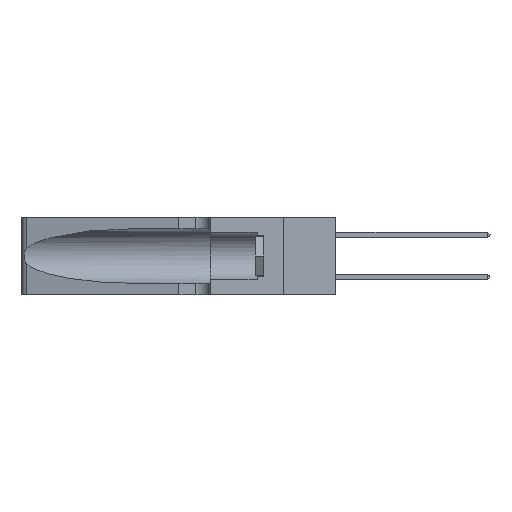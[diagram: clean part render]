
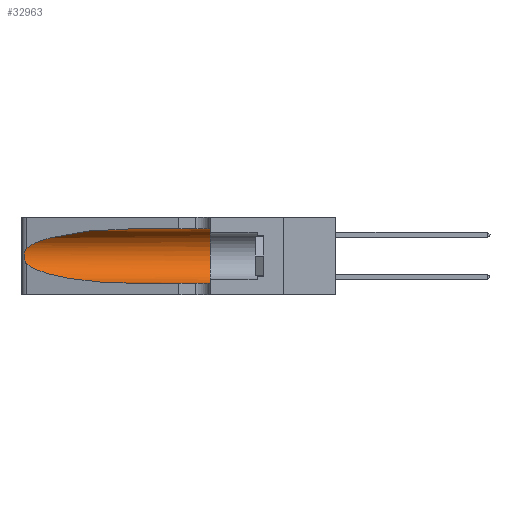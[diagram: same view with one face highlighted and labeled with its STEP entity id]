
A CAD part, left-side view. The second image highlights one B-rep face of the part: STEP entity #32963.
In plain terms, the highlighted cylindrical face has radius 3.308 mm (diameter 6.617 mm), a partial arc.
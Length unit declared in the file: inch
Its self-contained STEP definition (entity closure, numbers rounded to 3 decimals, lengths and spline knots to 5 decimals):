
#374 = EDGE_CURVE ( 'NONE', #2615, #19318, #17843, .T. ) ;
#410 = CARTESIAN_POINT ( 'NONE',  ( 0.18966, 0.96281, 0.05475 ) ) ;
#837 =( BOUNDED_CURVE ( )  B_SPLINE_CURVE ( 3, ( #3240, #30470, #410, #13938 ),
 .UNSPECIFIED., .F., .F. ) 
 B_SPLINE_CURVE_WITH_KNOTS ( ( 4, 4 ),
 ( 3.44316, 4.71239 ),
 .UNSPECIFIED. ) 
 CURVE ( )  GEOMETRIC_REPRESENTATION_ITEM ( )  RATIONAL_B_SPLINE_CURVE ( ( 1., 0.87, 0.87, 1. ) ) 
 REPRESENTATION_ITEM ( '' )  );
#1747 = CARTESIAN_POINT ( 'NONE',  ( 0.25487, 1.22718, 0.14631 ) ) ;
#2615 = VERTEX_POINT ( 'NONE', #20780 ) ;
#2907 = ORIENTED_EDGE ( 'NONE', *, *, #21805, .T. ) ;
#3240 = CARTESIAN_POINT ( 'NONE',  ( 0.25487, 1.22718, 0.14631 ) ) ;
#3848 = ORIENTED_EDGE ( 'NONE', *, *, #15714, .T. ) ;
#4164 = ORIENTED_EDGE ( 'NONE', *, *, #374, .F. ) ;
#4166 = CARTESIAN_POINT ( 'NONE',  ( 0.25555, 1.22994, 0.2215 ) ) ;
#4283 = CARTESIAN_POINT ( 'NONE',  ( 0.25639, 1.23186, 0.15144 ) ) ;
#5336 = CARTESIAN_POINT ( 'NONE',  ( 0.1305, 1.61858, 0.31525 ) ) ;
#5364 = LINE ( 'NONE', #10373, #8414 ) ;
#5399 = CARTESIAN_POINT ( 'NONE',  ( 0.1305, 0.72297, 0.31525 ) ) ;
#5685 = VERTEX_POINT ( 'NONE', #25413 ) ;
#6940 = CARTESIAN_POINT ( 'NONE',  ( 0.25555, 1.22993, 0.14849 ) ) ;
#7965 = LINE ( 'NONE', #5336, #10157 ) ;
#8414 = VECTOR ( 'NONE', #18704, 39.37008 ) ;
#8447 = CARTESIAN_POINT ( 'NONE',  ( 0.25487, 1.22718, 0.22369 ) ) ;
#10157 = VECTOR ( 'NONE', #19144, 39.37008 ) ;
#10373 = CARTESIAN_POINT ( 'NONE',  ( 0.1305, 1.61858, 0.05475 ) ) ;
#11327 = CARTESIAN_POINT ( 'NONE',  ( 0.1305, 0.35, 0.05475 ) ) ;
#11475 = AXIS2_PLACEMENT_3D ( 'NONE', #22306, #22669, #14192 ) ;
#11914 = B_SPLINE_CURVE_WITH_KNOTS ( 'NONE', 3,
 ( #15101, #4166, #31784, #15339, #20682, #23367, #12471, #34529, #17951, #18066, #20565, #4283, #6940, #1747 ),
 .UNSPECIFIED., .F., .F.,
 ( 4, 2, 2, 2, 2, 2, 4 ),
 ( 0., 0.00027, 0.00053, 0.00107, 0.0016, 0.00187, 0.00214 ),
 .UNSPECIFIED. ) ;
#12471 = CARTESIAN_POINT ( 'NONE',  ( 0.26075, 1.23896, 0.19203 ) ) ;
#13393 = CARTESIAN_POINT ( 'NONE',  ( 0.1305, 0.72297, 0.31525 ) ) ;
#13938 = CARTESIAN_POINT ( 'NONE',  ( 0.1305, 0.72297, 0.05475 ) ) ;
#14192 = DIRECTION ( 'NONE',  ( 0., 0., -1. ) ) ;
#14695 = CARTESIAN_POINT ( 'NONE',  ( 0.25487, 1.22718, 0.22369 ) ) ;
#15101 = CARTESIAN_POINT ( 'NONE',  ( 0.25487, 1.22718, 0.22369 ) ) ;
#15339 = CARTESIAN_POINT ( 'NONE',  ( 0.25787, 1.23484, 0.2124 ) ) ;
#15714 = EDGE_CURVE ( 'NONE', #22904, #5685, #11914, .T. ) ;
#17843 = CIRCLE ( 'NONE', #31739, 0.13025 ) ;
#17951 = CARTESIAN_POINT ( 'NONE',  ( 0.26017, 1.23833, 0.17102 ) ) ;
#18066 = CARTESIAN_POINT ( 'NONE',  ( 0.25856, 1.23593, 0.16098 ) ) ;
#18132 = CYLINDRICAL_SURFACE ( 'NONE', #11475, 0.13025 ) ;
#18673 = EDGE_CURVE ( 'NONE', #35394, #2615, #7965, .T. ) ;
#18704 = DIRECTION ( 'NONE',  ( 0., -1., 0. ) ) ;
#19015 = FACE_OUTER_BOUND ( 'NONE', #28119, .T. ) ;
#19144 = DIRECTION ( 'NONE',  ( 0., -1., 0. ) ) ;
#19318 = VERTEX_POINT ( 'NONE', #11327 ) ;
#20565 = CARTESIAN_POINT ( 'NONE',  ( 0.25789, 1.23486, 0.15765 ) ) ;
#20682 = CARTESIAN_POINT ( 'NONE',  ( 0.25854, 1.2359, 0.20912 ) ) ;
#20780 = CARTESIAN_POINT ( 'NONE',  ( 0.1305, 0.35, 0.31525 ) ) ;
#21805 = EDGE_CURVE ( 'NONE', #5685, #26155, #837, .T. ) ;
#22306 = CARTESIAN_POINT ( 'NONE',  ( 0.1305, 1.61858, 0.185 ) ) ;
#22669 = DIRECTION ( 'NONE',  ( 0., -1., 0. ) ) ;
#22904 = VERTEX_POINT ( 'NONE', #14695 ) ;
#23007 = CARTESIAN_POINT ( 'NONE',  ( 0.1305, 0.35, 0.185 ) ) ;
#23367 = CARTESIAN_POINT ( 'NONE',  ( 0.26018, 1.23835, 0.19895 ) ) ;
#24597 = CARTESIAN_POINT ( 'NONE',  ( 0.18966, 0.96281, 0.31525 ) ) ;
#25413 = CARTESIAN_POINT ( 'NONE',  ( 0.25487, 1.22718, 0.14631 ) ) ;
#25578 = EDGE_CURVE ( 'NONE', #26155, #19318, #5364, .T. ) ;
#25955 = DIRECTION ( 'NONE',  ( 0., 0., 1. ) ) ;
#26072 = ORIENTED_EDGE ( 'NONE', *, *, #18673, .F. ) ;
#26155 = VERTEX_POINT ( 'NONE', #30675 ) ;
#28119 = EDGE_LOOP ( 'NONE', ( #31471, #3848, #2907, #34337, #4164, #26072 ) ) ;
#30470 = CARTESIAN_POINT ( 'NONE',  ( 0.2373, 1.15595, 0.08982 ) ) ;
#30675 = CARTESIAN_POINT ( 'NONE',  ( 0.1305, 0.72297, 0.05475 ) ) ;
#31471 = ORIENTED_EDGE ( 'NONE', *, *, #32951, .T. ) ;
#31739 = AXIS2_PLACEMENT_3D ( 'NONE', #23007, #33096, #25955 ) ;
#31784 = CARTESIAN_POINT ( 'NONE',  ( 0.25639, 1.23184, 0.21858 ) ) ;
#32932 = CARTESIAN_POINT ( 'NONE',  ( 0.2373, 1.15595, 0.28018 ) ) ;
#32951 = EDGE_CURVE ( 'NONE', #35394, #22904, #33012, .T. ) ;
#32963 = ADVANCED_FACE ( 'NONE', ( #19015 ), #18132, .F. ) ;
#33012 =( BOUNDED_CURVE ( )  B_SPLINE_CURVE ( 3, ( #5399, #24597, #32932, #8447 ),
 .UNSPECIFIED., .F., .F. ) 
 B_SPLINE_CURVE_WITH_KNOTS ( ( 4, 4 ),
 ( 1.5708, 2.84003 ),
 .UNSPECIFIED. ) 
 CURVE ( )  GEOMETRIC_REPRESENTATION_ITEM ( )  RATIONAL_B_SPLINE_CURVE ( ( 1., 0.87, 0.87, 1. ) ) 
 REPRESENTATION_ITEM ( '' )  );
#33096 = DIRECTION ( 'NONE',  ( 0., 1., 0. ) ) ;
#34337 = ORIENTED_EDGE ( 'NONE', *, *, #25578, .T. ) ;
#34529 = CARTESIAN_POINT ( 'NONE',  ( 0.26075, 1.23896, 0.178 ) ) ;
#35394 = VERTEX_POINT ( 'NONE', #13393 ) ;
